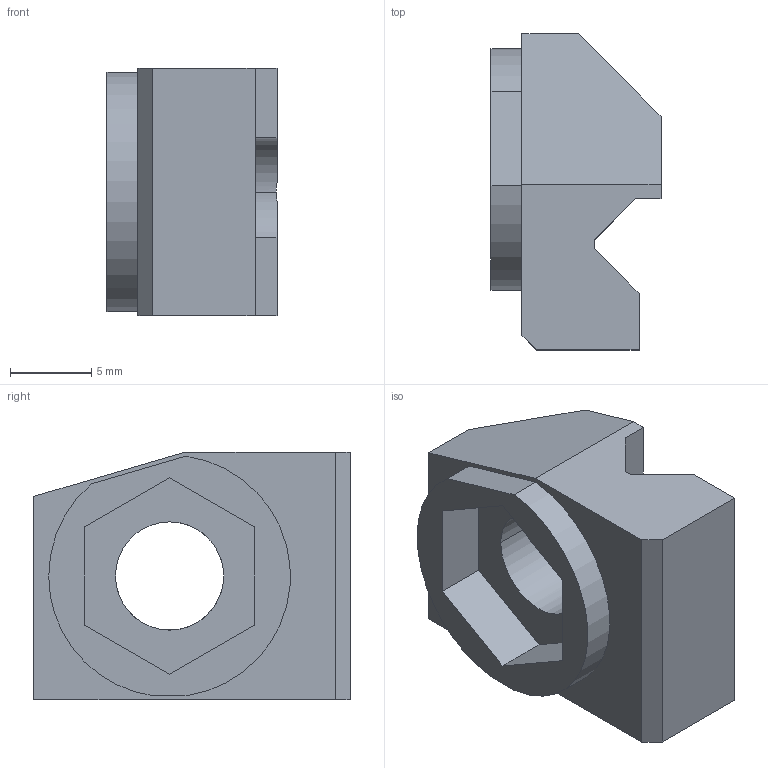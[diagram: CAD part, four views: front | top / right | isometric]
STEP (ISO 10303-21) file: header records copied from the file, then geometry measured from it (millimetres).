
FILE_DESCRIPTION (( 'STEP AP203' ), '1' );
FILE_NAME ('AF-WF-GS-PRT-002-STEP.STEP', '2020-07-21T19:00:38', ( '' ), ( '' ), 'SwSTEP 2.0', 'SolidWorks 2018', '' );
FILE_SCHEMA (( 'CONFIG_CONTROL_DESIGN' ));
Length unit declared in the file: inch
Products named in the file (1): AF-WF-GS-PRT-002-STEP
Bounding box: 10.47 x 19.48 x 15.24 mm (x, y, z)
Volume: 1712.8 mm3; surface area: 1323.4 mm2
Topology: 1 solids, 1 shells, 33 faces, 89 edges, 59 vertices
Faces by surface type: plane 28, cylinder 5
Entity records: 1109 total; most frequent: CARTESIAN_POINT 194, ORIENTED_EDGE 178, DIRECTION 164, EDGE_CURVE 89, VECTOR 74, LINE 74, VERTEX_POINT 59, AXIS2_PLACEMENT_3D 45
